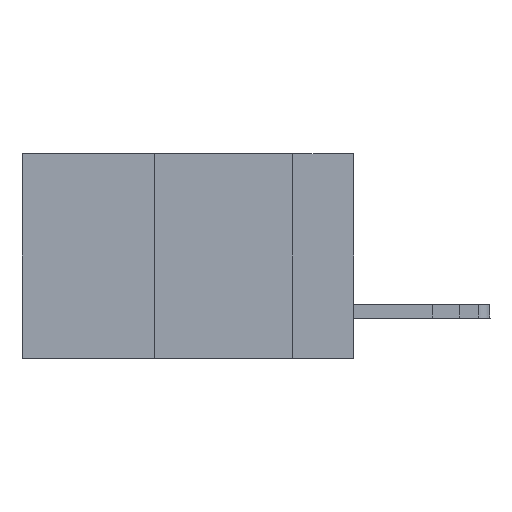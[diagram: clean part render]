
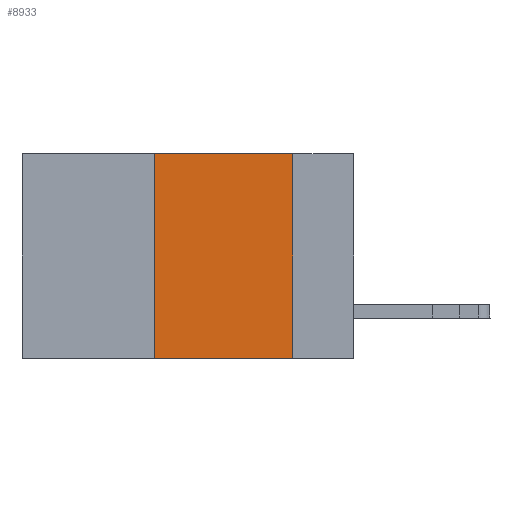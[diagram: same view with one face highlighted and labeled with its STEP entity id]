
A CAD part, left-side view. The second image highlights one B-rep face of the part: STEP entity #8933.
In plain terms, the highlighted planar face has unit normal (-1, 0, 0).
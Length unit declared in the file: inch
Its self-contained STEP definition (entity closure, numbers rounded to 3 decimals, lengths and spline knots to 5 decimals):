
#416 = VECTOR ( 'NONE', #7924, 39.37008 ) ;
#945 = AXIS2_PLACEMENT_3D ( 'NONE', #1665, #7234, #8898 ) ;
#1046 = ORIENTED_EDGE ( 'NONE', *, *, #11763, .F. ) ;
#1147 = CARTESIAN_POINT ( 'NONE',  ( 0., 0.36, 0. ) ) ;
#1307 = VECTOR ( 'NONE', #16430, 39.37008 ) ;
#1665 = CARTESIAN_POINT ( 'NONE',  ( 0., 0.6, 0. ) ) ;
#3125 = CARTESIAN_POINT ( 'NONE',  ( 0., 0.11, -0.37 ) ) ;
#3214 = VERTEX_POINT ( 'NONE', #3125 ) ;
#3795 = CARTESIAN_POINT ( 'NONE',  ( 0., 0.36, -0.37 ) ) ;
#7234 = DIRECTION ( 'NONE',  ( 1., 0., 0. ) ) ;
#7617 = CARTESIAN_POINT ( 'NONE',  ( 0., 0.11, 0. ) ) ;
#7854 = ORIENTED_EDGE ( 'NONE', *, *, #11325, .F. ) ;
#7924 = DIRECTION ( 'NONE',  ( 0., -1., 0. ) ) ;
#8898 = DIRECTION ( 'NONE',  ( 0., 0., -1. ) ) ;
#8933 = ADVANCED_FACE ( 'NONE', ( #21234 ), #15506, .F. ) ;
#9194 = LINE ( 'NONE', #7617, #1307 ) ;
#9484 = ORIENTED_EDGE ( 'NONE', *, *, #10368, .T. ) ;
#9942 = DIRECTION ( 'NONE',  ( 0., -1., 0. ) ) ;
#10368 = EDGE_CURVE ( 'NONE', #14183, #3214, #19550, .T. ) ;
#10772 = VERTEX_POINT ( 'NONE', #11805 ) ;
#11325 = EDGE_CURVE ( 'NONE', #21420, #10772, #18840, .T. ) ;
#11359 = LINE ( 'NONE', #1147, #17854 ) ;
#11763 = EDGE_CURVE ( 'NONE', #10772, #3214, #9194, .T. ) ;
#11805 = CARTESIAN_POINT ( 'NONE',  ( 0., 0.11, 0. ) ) ;
#11984 = VECTOR ( 'NONE', #9942, 39.37008 ) ;
#13617 = CARTESIAN_POINT ( 'NONE',  ( 0., 0.6, 0. ) ) ;
#14014 = CARTESIAN_POINT ( 'NONE',  ( 0., 0.36, 0. ) ) ;
#14183 = VERTEX_POINT ( 'NONE', #3795 ) ;
#14242 = EDGE_LOOP ( 'NONE', ( #1046, #7854, #16399, #9484 ) ) ;
#15506 = PLANE ( 'NONE',  #945 ) ;
#16399 = ORIENTED_EDGE ( 'NONE', *, *, #21753, .F. ) ;
#16430 = DIRECTION ( 'NONE',  ( 0., 0., -1. ) ) ;
#17854 = VECTOR ( 'NONE', #18484, 39.37008 ) ;
#18484 = DIRECTION ( 'NONE',  ( 0., 0., 1. ) ) ;
#18689 = CARTESIAN_POINT ( 'NONE',  ( 0., 0.6, -0.37 ) ) ;
#18840 = LINE ( 'NONE', #13617, #416 ) ;
#19550 = LINE ( 'NONE', #18689, #11984 ) ;
#21234 = FACE_OUTER_BOUND ( 'NONE', #14242, .T. ) ;
#21420 = VERTEX_POINT ( 'NONE', #14014 ) ;
#21753 = EDGE_CURVE ( 'NONE', #14183, #21420, #11359, .T. ) ;
